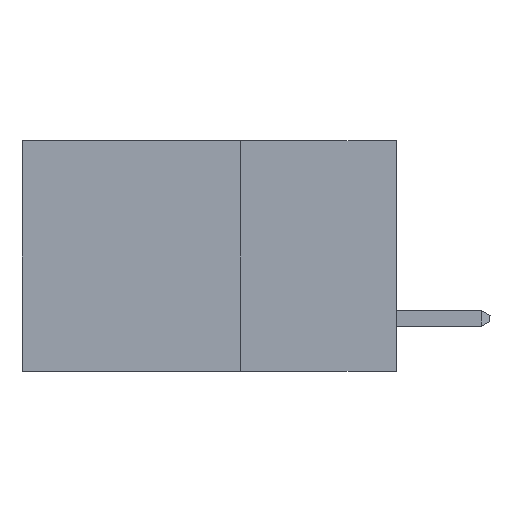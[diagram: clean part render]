
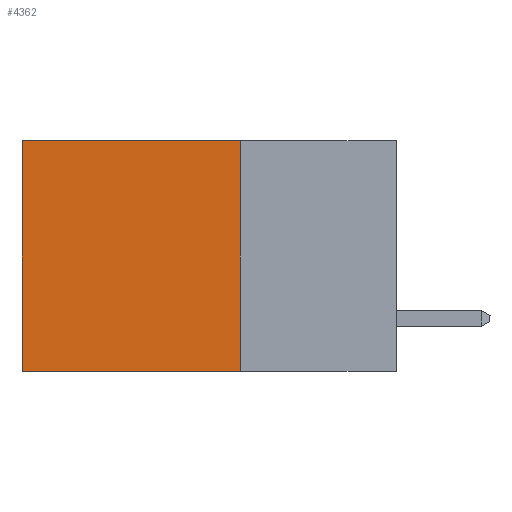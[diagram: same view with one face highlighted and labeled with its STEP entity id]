
A CAD part, left-side view. The second image highlights one B-rep face of the part: STEP entity #4362.
In plain terms, the highlighted planar face has unit normal (-1, 0, 0).
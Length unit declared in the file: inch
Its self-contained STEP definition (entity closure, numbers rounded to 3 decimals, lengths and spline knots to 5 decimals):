
#163 = CARTESIAN_POINT ( 'NONE',  ( 0.2615, 0.25, -0.37 ) ) ;
#251 = VERTEX_POINT ( 'NONE', #163 ) ;
#773 = ORIENTED_EDGE ( 'NONE', *, *, #11179, .T. ) ;
#892 = CARTESIAN_POINT ( 'NONE',  ( 0.2615, 0.6, -0.37 ) ) ;
#1067 = LINE ( 'NONE', #2504, #3470 ) ;
#1245 = DIRECTION ( 'NONE',  ( 1., 0., 0. ) ) ;
#1737 = CARTESIAN_POINT ( 'NONE',  ( 0.2615, 0.6, -0.37 ) ) ;
#2318 = FACE_OUTER_BOUND ( 'NONE', #14045, .T. ) ;
#2504 = CARTESIAN_POINT ( 'NONE',  ( 0.2615, 0.25, -0.37 ) ) ;
#2651 = VECTOR ( 'NONE', #11620, 39.37008 ) ;
#3470 = VECTOR ( 'NONE', #9863, 39.37008 ) ;
#3535 = PLANE ( 'NONE',  #12875 ) ;
#3764 = LINE ( 'NONE', #10337, #2651 ) ;
#3766 = EDGE_CURVE ( 'NONE', #10277, #251, #9091, .T. ) ;
#4362 = ADVANCED_FACE ( 'NONE', ( #2318 ), #3535, .F. ) ;
#5019 = EDGE_CURVE ( 'NONE', #251, #13834, #1067, .T. ) ;
#5253 = ORIENTED_EDGE ( 'NONE', *, *, #5019, .F. ) ;
#7605 = VECTOR ( 'NONE', #8091, 39.37008 ) ;
#7965 = VERTEX_POINT ( 'NONE', #9317 ) ;
#8091 = DIRECTION ( 'NONE',  ( 0., 0., -1. ) ) ;
#8965 = CARTESIAN_POINT ( 'NONE',  ( 0.2615, 0.25, -0.37 ) ) ;
#9091 = LINE ( 'NONE', #10234, #7605 ) ;
#9317 = CARTESIAN_POINT ( 'NONE',  ( 0.2615, 0.6, 0. ) ) ;
#9863 = DIRECTION ( 'NONE',  ( 0., 1., 0. ) ) ;
#10228 = CARTESIAN_POINT ( 'NONE',  ( 0.2615, 0.25, 0. ) ) ;
#10234 = CARTESIAN_POINT ( 'NONE',  ( 0.2615, 0.25, -0.37 ) ) ;
#10268 = ORIENTED_EDGE ( 'NONE', *, *, #3766, .F. ) ;
#10277 = VERTEX_POINT ( 'NONE', #10228 ) ;
#10337 = CARTESIAN_POINT ( 'NONE',  ( 0.2615, 0.25, 0. ) ) ;
#10917 = VECTOR ( 'NONE', #11978, 39.37008 ) ;
#11179 = EDGE_CURVE ( 'NONE', #10277, #7965, #3764, .T. ) ;
#11620 = DIRECTION ( 'NONE',  ( 0., 1., 0. ) ) ;
#11978 = DIRECTION ( 'NONE',  ( 0., 0., -1. ) ) ;
#12116 = DIRECTION ( 'NONE',  ( 0., 0., -1. ) ) ;
#12704 = EDGE_CURVE ( 'NONE', #7965, #13834, #13983, .T. ) ;
#12875 = AXIS2_PLACEMENT_3D ( 'NONE', #8965, #1245, #12116 ) ;
#12993 = ORIENTED_EDGE ( 'NONE', *, *, #12704, .T. ) ;
#13834 = VERTEX_POINT ( 'NONE', #1737 ) ;
#13983 = LINE ( 'NONE', #892, #10917 ) ;
#14045 = EDGE_LOOP ( 'NONE', ( #12993, #5253, #10268, #773 ) ) ;
